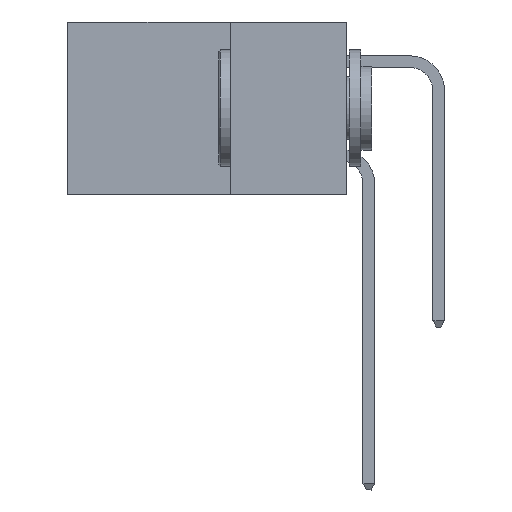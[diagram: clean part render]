
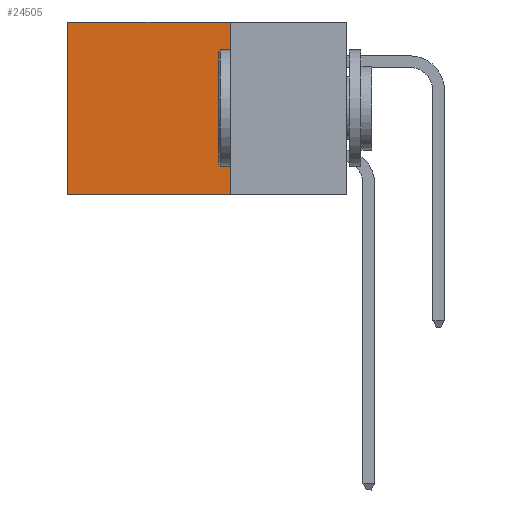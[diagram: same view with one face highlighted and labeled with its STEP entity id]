
A CAD part, left-side view. The second image highlights one B-rep face of the part: STEP entity #24505.
In plain terms, the highlighted planar face has unit normal (-1, 0, 0).
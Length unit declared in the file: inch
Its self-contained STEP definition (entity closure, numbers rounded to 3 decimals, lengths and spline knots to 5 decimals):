
#213 = ORIENTED_EDGE ( 'NONE', *, *, #13239, .T. ) ;
#803 = EDGE_LOOP ( 'NONE', ( #213, #41801, #9875, #33175 ) ) ;
#2099 = LINE ( 'NONE', #26471, #37446 ) ;
#3577 = LINE ( 'NONE', #12487, #11870 ) ;
#6357 = VERTEX_POINT ( 'NONE', #9835 ) ;
#9534 = PLANE ( 'NONE',  #28131 ) ;
#9835 = CARTESIAN_POINT ( 'NONE',  ( 0.2875, 0.25, -0.37 ) ) ;
#9875 = ORIENTED_EDGE ( 'NONE', *, *, #11772, .F. ) ;
#10062 = CARTESIAN_POINT ( 'NONE',  ( 0.2875, 0.6, -0.37 ) ) ;
#11772 = EDGE_CURVE ( 'NONE', #12885, #6357, #2099, .T. ) ;
#11870 = VECTOR ( 'NONE', #40441, 39.37008 ) ;
#11886 = CARTESIAN_POINT ( 'NONE',  ( 0.2875, 0.25, -0.37 ) ) ;
#12487 = CARTESIAN_POINT ( 'NONE',  ( 0.2875, 0.6, 0. ) ) ;
#12885 = VERTEX_POINT ( 'NONE', #13582 ) ;
#12929 = LINE ( 'NONE', #34709, #14063 ) ;
#13239 = EDGE_CURVE ( 'NONE', #30863, #14133, #3577, .T. ) ;
#13582 = CARTESIAN_POINT ( 'NONE',  ( 0.2875, 0.25, 0. ) ) ;
#13583 = EDGE_CURVE ( 'NONE', #12885, #30863, #12929, .T. ) ;
#14063 = VECTOR ( 'NONE', #45333, 39.37008 ) ;
#14133 = VERTEX_POINT ( 'NONE', #10062 ) ;
#16113 = DIRECTION ( 'NONE',  ( 0., 0., -1. ) ) ;
#16613 = DIRECTION ( 'NONE',  ( 1., 0., 0. ) ) ;
#19845 = DIRECTION ( 'NONE',  ( 0., 0., -1. ) ) ;
#21790 = LINE ( 'NONE', #11886, #36169 ) ;
#22496 = FACE_OUTER_BOUND ( 'NONE', #803, .T. ) ;
#22673 = DIRECTION ( 'NONE',  ( 0., 1., 0. ) ) ;
#24505 = ADVANCED_FACE ( 'NONE', ( #22496 ), #9534, .F. ) ;
#26471 = CARTESIAN_POINT ( 'NONE',  ( 0.2875, 0.25, 0. ) ) ;
#28131 = AXIS2_PLACEMENT_3D ( 'NONE', #30972, #16613, #19845 ) ;
#29870 = CARTESIAN_POINT ( 'NONE',  ( 0.2875, 0.6, 0. ) ) ;
#30863 = VERTEX_POINT ( 'NONE', #29870 ) ;
#30972 = CARTESIAN_POINT ( 'NONE',  ( 0.2875, 0.25, 0. ) ) ;
#33175 = ORIENTED_EDGE ( 'NONE', *, *, #13583, .T. ) ;
#34709 = CARTESIAN_POINT ( 'NONE',  ( 0.2875, 0.25, 0. ) ) ;
#36169 = VECTOR ( 'NONE', #22673, 39.37008 ) ;
#37446 = VECTOR ( 'NONE', #16113, 39.37008 ) ;
#40441 = DIRECTION ( 'NONE',  ( 0., 0., -1. ) ) ;
#41753 = EDGE_CURVE ( 'NONE', #6357, #14133, #21790, .T. ) ;
#41801 = ORIENTED_EDGE ( 'NONE', *, *, #41753, .F. ) ;
#45333 = DIRECTION ( 'NONE',  ( 0., 1., 0. ) ) ;
